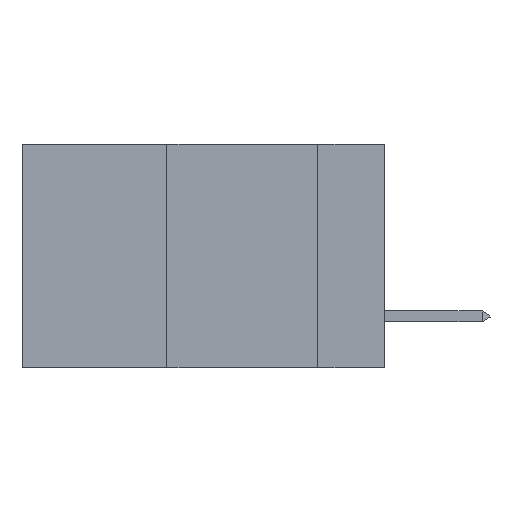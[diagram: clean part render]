
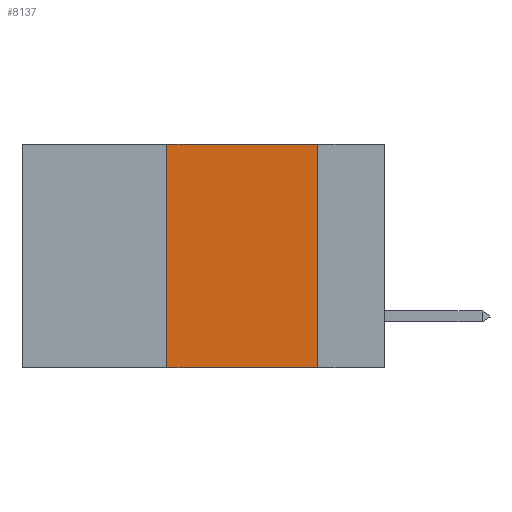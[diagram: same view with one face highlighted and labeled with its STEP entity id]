
A CAD part, left-side view. The second image highlights one B-rep face of the part: STEP entity #8137.
In plain terms, the highlighted planar face has unit normal (-1, 0, 0).
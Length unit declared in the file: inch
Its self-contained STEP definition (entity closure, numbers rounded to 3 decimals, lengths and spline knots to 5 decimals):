
#1307 = CARTESIAN_POINT ( 'NONE',  ( 0., 0.36, -0.37 ) ) ;
#1544 = VECTOR ( 'NONE', #13773, 39.37008 ) ;
#1766 = CARTESIAN_POINT ( 'NONE',  ( 0., 0.36, 0. ) ) ;
#2802 = DIRECTION ( 'NONE',  ( 0., 0., 1. ) ) ;
#3546 = ORIENTED_EDGE ( 'NONE', *, *, #8812, .F. ) ;
#4351 = DIRECTION ( 'NONE',  ( 1., 0., 0. ) ) ;
#4943 = VECTOR ( 'NONE', #6059, 39.37008 ) ;
#5130 = CARTESIAN_POINT ( 'NONE',  ( 0., 0.11, 0. ) ) ;
#6059 = DIRECTION ( 'NONE',  ( 0., -1., 0. ) ) ;
#7494 = CARTESIAN_POINT ( 'NONE',  ( 0., 0.6, 0. ) ) ;
#8137 = ADVANCED_FACE ( 'NONE', ( #10088 ), #15021, .F. ) ;
#8259 = VERTEX_POINT ( 'NONE', #1766 ) ;
#8812 = EDGE_CURVE ( 'NONE', #13601, #8259, #15700, .T. ) ;
#9729 = EDGE_CURVE ( 'NONE', #13601, #11065, #10530, .T. ) ;
#10088 = FACE_OUTER_BOUND ( 'NONE', #19250, .T. ) ;
#10530 = LINE ( 'NONE', #16874, #4943 ) ;
#10848 = CARTESIAN_POINT ( 'NONE',  ( 0., 0.11, 0. ) ) ;
#11065 = VERTEX_POINT ( 'NONE', #15941 ) ;
#11565 = VECTOR ( 'NONE', #2802, 39.37008 ) ;
#11648 = EDGE_CURVE ( 'NONE', #18153, #11065, #19446, .T. ) ;
#11692 = AXIS2_PLACEMENT_3D ( 'NONE', #7494, #4351, #11901 ) ;
#11901 = DIRECTION ( 'NONE',  ( 0., 0., -1. ) ) ;
#13086 = EDGE_CURVE ( 'NONE', #8259, #18153, #17300, .T. ) ;
#13601 = VERTEX_POINT ( 'NONE', #1307 ) ;
#13773 = DIRECTION ( 'NONE',  ( 0., -1., 0. ) ) ;
#13893 = ORIENTED_EDGE ( 'NONE', *, *, #11648, .F. ) ;
#13920 = DIRECTION ( 'NONE',  ( 0., 0., -1. ) ) ;
#14511 = ORIENTED_EDGE ( 'NONE', *, *, #13086, .F. ) ;
#15021 = PLANE ( 'NONE',  #11692 ) ;
#15498 = CARTESIAN_POINT ( 'NONE',  ( 0., 0.6, 0. ) ) ;
#15593 = VECTOR ( 'NONE', #13920, 39.37008 ) ;
#15700 = LINE ( 'NONE', #19662, #11565 ) ;
#15941 = CARTESIAN_POINT ( 'NONE',  ( 0., 0.11, -0.37 ) ) ;
#16528 = ORIENTED_EDGE ( 'NONE', *, *, #9729, .T. ) ;
#16874 = CARTESIAN_POINT ( 'NONE',  ( 0., 0.6, -0.37 ) ) ;
#17300 = LINE ( 'NONE', #15498, #1544 ) ;
#18153 = VERTEX_POINT ( 'NONE', #5130 ) ;
#19250 = EDGE_LOOP ( 'NONE', ( #13893, #14511, #3546, #16528 ) ) ;
#19446 = LINE ( 'NONE', #10848, #15593 ) ;
#19662 = CARTESIAN_POINT ( 'NONE',  ( 0., 0.36, 0. ) ) ;
